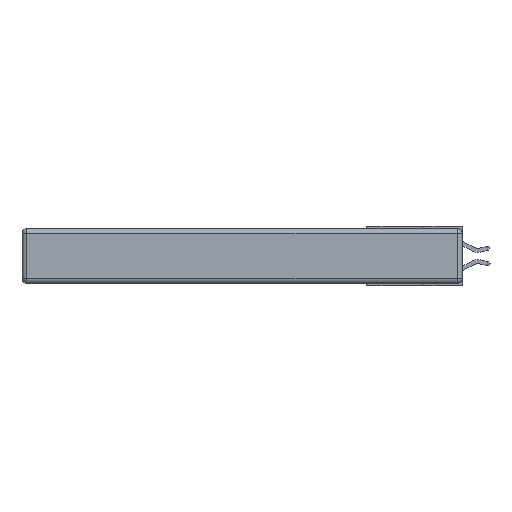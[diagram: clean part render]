
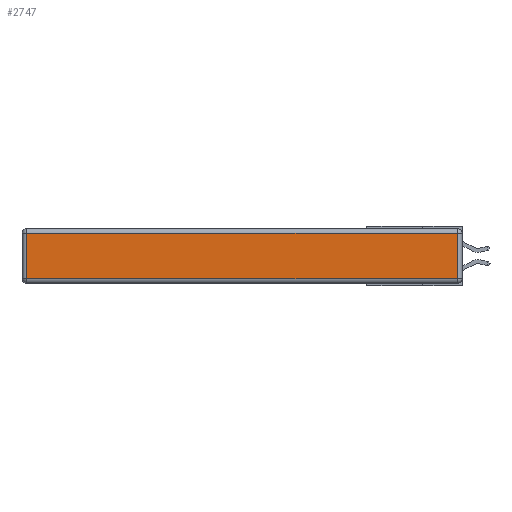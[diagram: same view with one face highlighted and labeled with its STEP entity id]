
A CAD part, left-side view. The second image highlights one B-rep face of the part: STEP entity #2747.
In plain terms, the highlighted planar face has unit normal (-1, 0, 0).
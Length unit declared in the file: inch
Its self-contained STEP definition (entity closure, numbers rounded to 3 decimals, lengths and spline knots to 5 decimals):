
#513 = CARTESIAN_POINT ( 'NONE',  ( 0., 0., -0.343 ) ) ;
#817 = CARTESIAN_POINT ( 'NONE',  ( 0., 2.72, -0.03 ) ) ;
#1187 = ORIENTED_EDGE ( 'NONE', *, *, #13263, .T. ) ;
#1626 = DIRECTION ( 'NONE',  ( 0., 0., 1. ) ) ;
#1842 = ORIENTED_EDGE ( 'NONE', *, *, #13145, .T. ) ;
#1897 = CARTESIAN_POINT ( 'NONE',  ( 0., 2.75, -0.03 ) ) ;
#2216 = CARTESIAN_POINT ( 'NONE',  ( 0., 0.03, -0.343 ) ) ;
#2747 = ADVANCED_FACE ( 'NONE', ( #12680 ), #6817, .T. ) ;
#3387 = CARTESIAN_POINT ( 'NONE',  ( 0., 2.72, -0.343 ) ) ;
#3431 = VECTOR ( 'NONE', #9858, 39.37008 ) ;
#3559 = EDGE_CURVE ( 'NONE', #4712, #4728, #4572, .T. ) ;
#3852 = CARTESIAN_POINT ( 'NONE',  ( 0., 0.03, -0.03 ) ) ;
#3933 = LINE ( 'NONE', #2216, #10022 ) ;
#4383 = DIRECTION ( 'NONE',  ( 0., 0., 1. ) ) ;
#4510 = DIRECTION ( 'NONE',  ( 0., 0., -1. ) ) ;
#4572 = LINE ( 'NONE', #1897, #9495 ) ;
#4712 = VERTEX_POINT ( 'NONE', #3852 ) ;
#4728 = VERTEX_POINT ( 'NONE', #817 ) ;
#5400 = LINE ( 'NONE', #8796, #3431 ) ;
#6817 = PLANE ( 'NONE',  #9165 ) ;
#7405 = VECTOR ( 'NONE', #4510, 39.37008 ) ;
#8796 = CARTESIAN_POINT ( 'NONE',  ( 0., 0., -0.313 ) ) ;
#9165 = AXIS2_PLACEMENT_3D ( 'NONE', #513, #11038, #1626 ) ;
#9373 = ORIENTED_EDGE ( 'NONE', *, *, #3559, .T. ) ;
#9458 = CARTESIAN_POINT ( 'NONE',  ( 0., 0.03, -0.313 ) ) ;
#9495 = VECTOR ( 'NONE', #12411, 39.37008 ) ;
#9858 = DIRECTION ( 'NONE',  ( 0., -1., 0. ) ) ;
#10022 = VECTOR ( 'NONE', #4383, 39.37008 ) ;
#10461 = VERTEX_POINT ( 'NONE', #12875 ) ;
#11038 = DIRECTION ( 'NONE',  ( -1., 0., 0. ) ) ;
#11152 = ORIENTED_EDGE ( 'NONE', *, *, #11662, .T. ) ;
#11662 = EDGE_CURVE ( 'NONE', #4728, #10461, #13475, .T. ) ;
#11816 = EDGE_LOOP ( 'NONE', ( #1187, #1842, #9373, #11152 ) ) ;
#12411 = DIRECTION ( 'NONE',  ( 0., 1., 0. ) ) ;
#12680 = FACE_OUTER_BOUND ( 'NONE', #11816, .T. ) ;
#12875 = CARTESIAN_POINT ( 'NONE',  ( 0., 2.72, -0.313 ) ) ;
#13145 = EDGE_CURVE ( 'NONE', #13584, #4712, #3933, .T. ) ;
#13263 = EDGE_CURVE ( 'NONE', #10461, #13584, #5400, .T. ) ;
#13475 = LINE ( 'NONE', #3387, #7405 ) ;
#13584 = VERTEX_POINT ( 'NONE', #9458 ) ;
